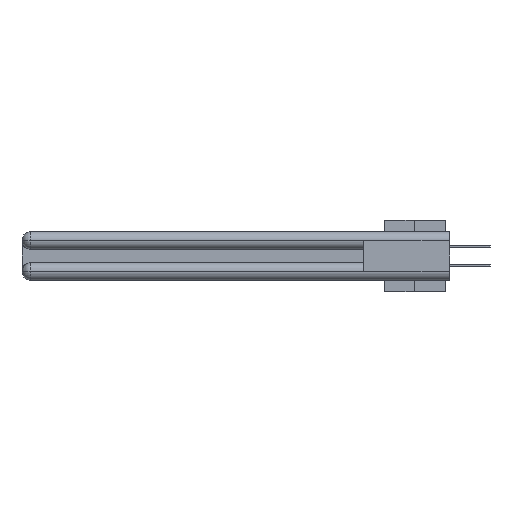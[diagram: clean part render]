
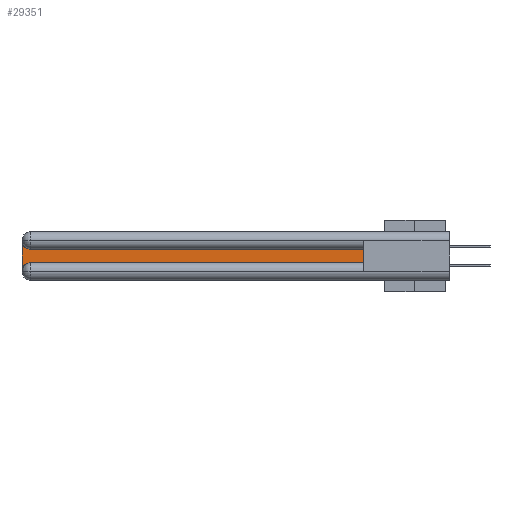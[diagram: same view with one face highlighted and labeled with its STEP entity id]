
A CAD part, left-side view. The second image highlights one B-rep face of the part: STEP entity #29351.
In plain terms, the highlighted planar face has unit normal (-1, 0, 0).
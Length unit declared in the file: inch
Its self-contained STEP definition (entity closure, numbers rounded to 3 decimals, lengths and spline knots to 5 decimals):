
#95 = VECTOR ( 'NONE', #8921, 39.37008 ) ;
#1156 = DIRECTION ( 'NONE',  ( 1., 0., 0. ) ) ;
#1867 = CARTESIAN_POINT ( 'NONE',  ( 0.075, 0.6, -0.2175 ) ) ;
#1969 = ORIENTED_EDGE ( 'NONE', *, *, #40394, .T. ) ;
#2685 = DIRECTION ( 'NONE',  ( 0., 0., 1. ) ) ;
#3293 = EDGE_CURVE ( 'NONE', #24952, #33449, #17155, .T. ) ;
#4315 = EDGE_CURVE ( 'NONE', #13859, #8091, #16805, .T. ) ;
#5029 = AXIS2_PLACEMENT_3D ( 'NONE', #18735, #44157, #22396 ) ;
#6066 = CARTESIAN_POINT ( 'NONE',  ( 0.075, 0.6, -0.2175 ) ) ;
#7291 = CIRCLE ( 'NONE', #15808, 0.06 ) ;
#7743 = CARTESIAN_POINT ( 'NONE',  ( 0.075, 2.94, -0.1225 ) ) ;
#8091 = VERTEX_POINT ( 'NONE', #33989 ) ;
#8556 = EDGE_CURVE ( 'NONE', #33449, #28909, #7291, .T. ) ;
#8921 = DIRECTION ( 'NONE',  ( 0., 1., 0. ) ) ;
#9186 = LINE ( 'NONE', #19752, #10853 ) ;
#9409 = CARTESIAN_POINT ( 'NONE',  ( 0.075, 2.94, -0.0625 ) ) ;
#10467 = VECTOR ( 'NONE', #2685, 39.37008 ) ;
#10853 = VECTOR ( 'NONE', #45233, 39.37008 ) ;
#12682 = CARTESIAN_POINT ( 'NONE',  ( 0.075, 0.6, -0.2175 ) ) ;
#13859 = VERTEX_POINT ( 'NONE', #16241 ) ;
#14666 = ORIENTED_EDGE ( 'NONE', *, *, #14988, .T. ) ;
#14873 = CARTESIAN_POINT ( 'NONE',  ( 0.075, 3., -0.1225 ) ) ;
#14988 = EDGE_CURVE ( 'NONE', #28909, #13859, #9186, .T. ) ;
#15808 = AXIS2_PLACEMENT_3D ( 'NONE', #9409, #1156, #44914 ) ;
#16241 = CARTESIAN_POINT ( 'NONE',  ( 0.075, 3., -0.2775 ) ) ;
#16267 = LINE ( 'NONE', #1867, #45352 ) ;
#16805 = CIRCLE ( 'NONE', #5029, 0.06 ) ;
#17155 = LINE ( 'NONE', #23413, #95 ) ;
#17552 = ORIENTED_EDGE ( 'NONE', *, *, #4315, .T. ) ;
#18735 = CARTESIAN_POINT ( 'NONE',  ( 0.075, 2.94, -0.2775 ) ) ;
#19752 = CARTESIAN_POINT ( 'NONE',  ( 0.075, 3., -0.2175 ) ) ;
#21299 = LINE ( 'NONE', #6066, #10467 ) ;
#22142 = FACE_OUTER_BOUND ( 'NONE', #25818, .T. ) ;
#22396 = DIRECTION ( 'NONE',  ( 0., 0., -1. ) ) ;
#22622 = CARTESIAN_POINT ( 'NONE',  ( 0.075, 3., -0.0625 ) ) ;
#23413 = CARTESIAN_POINT ( 'NONE',  ( 0.075, 0.6, -0.1225 ) ) ;
#23986 = DIRECTION ( 'NONE',  ( 0., -1., 0. ) ) ;
#24952 = VERTEX_POINT ( 'NONE', #30899 ) ;
#25818 = EDGE_LOOP ( 'NONE', ( #38251, #36510, #14666, #17552, #1969, #34657 ) ) ;
#28909 = VERTEX_POINT ( 'NONE', #22622 ) ;
#29351 = ADVANCED_FACE ( 'NONE', ( #22142 ), #29864, .F. ) ;
#29864 = PLANE ( 'NONE',  #43328 ) ;
#30899 = CARTESIAN_POINT ( 'NONE',  ( 0.075, 0.6, -0.1225 ) ) ;
#32193 = EDGE_CURVE ( 'NONE', #41883, #24952, #21299, .T. ) ;
#33449 = VERTEX_POINT ( 'NONE', #7743 ) ;
#33989 = CARTESIAN_POINT ( 'NONE',  ( 0.075, 2.94, -0.2175 ) ) ;
#34657 = ORIENTED_EDGE ( 'NONE', *, *, #32193, .T. ) ;
#36491 = DIRECTION ( 'NONE',  ( 0., 0., -1. ) ) ;
#36510 = ORIENTED_EDGE ( 'NONE', *, *, #8556, .T. ) ;
#36985 = DIRECTION ( 'NONE',  ( 1., 0., 0. ) ) ;
#38251 = ORIENTED_EDGE ( 'NONE', *, *, #3293, .T. ) ;
#40394 = EDGE_CURVE ( 'NONE', #8091, #41883, #16267, .T. ) ;
#41883 = VERTEX_POINT ( 'NONE', #12682 ) ;
#43328 = AXIS2_PLACEMENT_3D ( 'NONE', #14873, #36985, #36491 ) ;
#44157 = DIRECTION ( 'NONE',  ( 1., 0., 0. ) ) ;
#44914 = DIRECTION ( 'NONE',  ( 0., 0., -1. ) ) ;
#45233 = DIRECTION ( 'NONE',  ( 0., 0., -1. ) ) ;
#45352 = VECTOR ( 'NONE', #23986, 39.37008 ) ;
